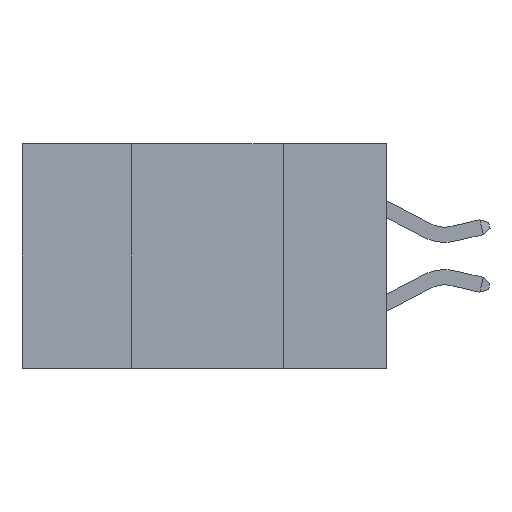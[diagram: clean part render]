
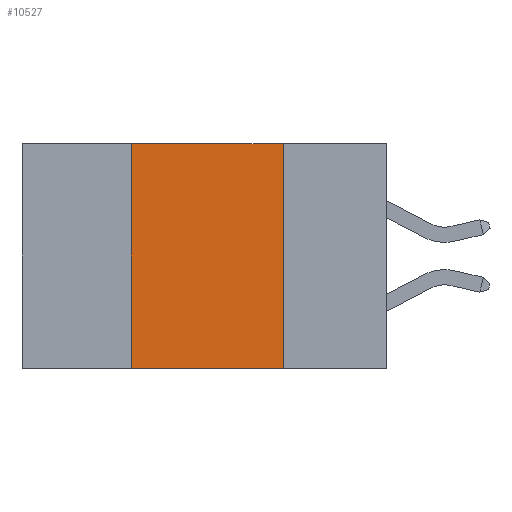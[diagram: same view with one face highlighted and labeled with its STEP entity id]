
A CAD part, left-side view. The second image highlights one B-rep face of the part: STEP entity #10527.
In plain terms, the highlighted planar face has unit normal (-1, 0, 0).
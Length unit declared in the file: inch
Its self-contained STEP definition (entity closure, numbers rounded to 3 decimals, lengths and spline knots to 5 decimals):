
#450 = EDGE_CURVE ( 'NONE', #10423, #1627, #10143, .T. ) ;
#664 = VECTOR ( 'NONE', #9326, 39.37008 ) ;
#1100 = DIRECTION ( 'NONE',  ( 0., -1., 0. ) ) ;
#1627 = VERTEX_POINT ( 'NONE', #5675 ) ;
#1919 = EDGE_CURVE ( 'NONE', #10423, #7509, #3812, .T. ) ;
#1932 = DIRECTION ( 'NONE',  ( 0., 0., -1. ) ) ;
#1984 = ORIENTED_EDGE ( 'NONE', *, *, #12058, .F. ) ;
#2121 = ORIENTED_EDGE ( 'NONE', *, *, #2646, .F. ) ;
#2268 = ORIENTED_EDGE ( 'NONE', *, *, #450, .F. ) ;
#2423 = ORIENTED_EDGE ( 'NONE', *, *, #1919, .T. ) ;
#2488 = AXIS2_PLACEMENT_3D ( 'NONE', #6865, #8995, #2662 ) ;
#2646 = EDGE_CURVE ( 'NONE', #1627, #5897, #3832, .T. ) ;
#2662 = DIRECTION ( 'NONE',  ( 0., 0., -1. ) ) ;
#2905 = EDGE_LOOP ( 'NONE', ( #1984, #2121, #2268, #2423 ) ) ;
#3812 = LINE ( 'NONE', #10940, #9099 ) ;
#3832 = LINE ( 'NONE', #6982, #664 ) ;
#5074 = CARTESIAN_POINT ( 'NONE',  ( 0., 0.17, 0. ) ) ;
#5103 = VECTOR ( 'NONE', #1932, 39.37008 ) ;
#5607 = CARTESIAN_POINT ( 'NONE',  ( 0., 0.17, 0. ) ) ;
#5675 = CARTESIAN_POINT ( 'NONE',  ( 0., 0.42, 0. ) ) ;
#5897 = VERTEX_POINT ( 'NONE', #5607 ) ;
#6865 = CARTESIAN_POINT ( 'NONE',  ( 0., 0.6, 0. ) ) ;
#6982 = CARTESIAN_POINT ( 'NONE',  ( 0., 0.6, 0. ) ) ;
#7509 = VERTEX_POINT ( 'NONE', #7909 ) ;
#7909 = CARTESIAN_POINT ( 'NONE',  ( 0., 0.17, -0.37 ) ) ;
#7927 = LINE ( 'NONE', #5074, #5103 ) ;
#7943 = PLANE ( 'NONE',  #2488 ) ;
#8706 = CARTESIAN_POINT ( 'NONE',  ( 0., 0.42, 0. ) ) ;
#8995 = DIRECTION ( 'NONE',  ( 1., 0., 0. ) ) ;
#9099 = VECTOR ( 'NONE', #1100, 39.37008 ) ;
#9231 = DIRECTION ( 'NONE',  ( 0., 0., 1. ) ) ;
#9326 = DIRECTION ( 'NONE',  ( 0., -1., 0. ) ) ;
#9811 = VECTOR ( 'NONE', #9231, 39.37008 ) ;
#10143 = LINE ( 'NONE', #8706, #9811 ) ;
#10423 = VERTEX_POINT ( 'NONE', #10984 ) ;
#10527 = ADVANCED_FACE ( 'NONE', ( #10946 ), #7943, .F. ) ;
#10940 = CARTESIAN_POINT ( 'NONE',  ( 0., 0.6, -0.37 ) ) ;
#10946 = FACE_OUTER_BOUND ( 'NONE', #2905, .T. ) ;
#10984 = CARTESIAN_POINT ( 'NONE',  ( 0., 0.42, -0.37 ) ) ;
#12058 = EDGE_CURVE ( 'NONE', #5897, #7509, #7927, .T. ) ;
